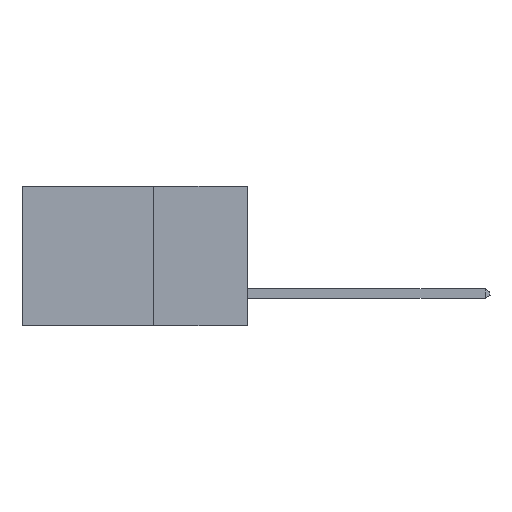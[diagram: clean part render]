
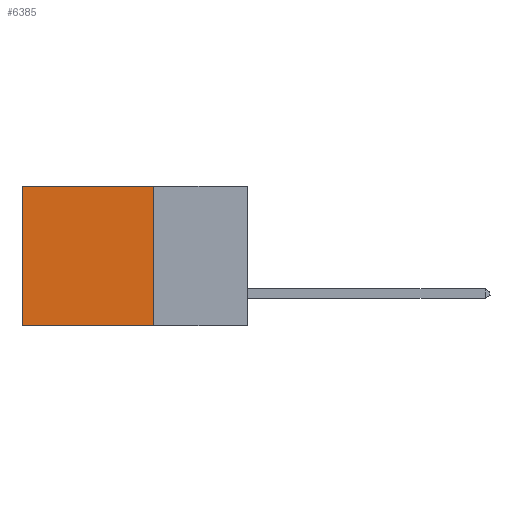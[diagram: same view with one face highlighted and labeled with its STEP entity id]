
A CAD part, left-side view. The second image highlights one B-rep face of the part: STEP entity #6385.
In plain terms, the highlighted planar face has unit normal (-1, 0, 0).
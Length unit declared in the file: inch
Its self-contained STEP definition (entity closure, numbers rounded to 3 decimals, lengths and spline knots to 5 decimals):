
#765 = ORIENTED_EDGE ( 'NONE', *, *, #7587, .F. ) ;
#781 = CARTESIAN_POINT ( 'NONE',  ( 0.298, 0.6, 0. ) ) ;
#1772 = LINE ( 'NONE', #2272, #2095 ) ;
#1887 = DIRECTION ( 'NONE',  ( 1., 0., 0. ) ) ;
#1901 = ORIENTED_EDGE ( 'NONE', *, *, #11786, .T. ) ;
#1933 = DIRECTION ( 'NONE',  ( 0., 0., -1. ) ) ;
#1983 = LINE ( 'NONE', #12808, #10273 ) ;
#2095 = VECTOR ( 'NONE', #10587, 39.37008 ) ;
#2272 = CARTESIAN_POINT ( 'NONE',  ( 0.298, 0.25, 0. ) ) ;
#2863 = AXIS2_PLACEMENT_3D ( 'NONE', #11199, #1887, #1933 ) ;
#2880 = CARTESIAN_POINT ( 'NONE',  ( 0.298, 0.25, -0.37 ) ) ;
#3035 = CARTESIAN_POINT ( 'NONE',  ( 0.298, 0.25, -0.37 ) ) ;
#3577 = CARTESIAN_POINT ( 'NONE',  ( 0.298, 0.6, -0.37 ) ) ;
#3998 = PLANE ( 'NONE',  #2863 ) ;
#4485 = DIRECTION ( 'NONE',  ( 0., 1., 0. ) ) ;
#4574 = VERTEX_POINT ( 'NONE', #5462 ) ;
#4881 = EDGE_LOOP ( 'NONE', ( #1901, #8925, #765, #7306 ) ) ;
#5462 = CARTESIAN_POINT ( 'NONE',  ( 0.298, 0.6, 0. ) ) ;
#5832 = EDGE_CURVE ( 'NONE', #10118, #4574, #1983, .T. ) ;
#5846 = DIRECTION ( 'NONE',  ( 0., 1., 0. ) ) ;
#5921 = VERTEX_POINT ( 'NONE', #3577 ) ;
#6385 = ADVANCED_FACE ( 'NONE', ( #7157 ), #3998, .F. ) ;
#7157 = FACE_OUTER_BOUND ( 'NONE', #4881, .T. ) ;
#7306 = ORIENTED_EDGE ( 'NONE', *, *, #5832, .T. ) ;
#7587 = EDGE_CURVE ( 'NONE', #10118, #10417, #1772, .T. ) ;
#7695 = LINE ( 'NONE', #2880, #10621 ) ;
#8031 = DIRECTION ( 'NONE',  ( 0., 0., -1. ) ) ;
#8925 = ORIENTED_EDGE ( 'NONE', *, *, #10825, .F. ) ;
#9440 = CARTESIAN_POINT ( 'NONE',  ( 0.298, 0.25, 0. ) ) ;
#9574 = VECTOR ( 'NONE', #8031, 39.37008 ) ;
#10118 = VERTEX_POINT ( 'NONE', #9440 ) ;
#10273 = VECTOR ( 'NONE', #4485, 39.37008 ) ;
#10417 = VERTEX_POINT ( 'NONE', #3035 ) ;
#10587 = DIRECTION ( 'NONE',  ( 0., 0., -1. ) ) ;
#10621 = VECTOR ( 'NONE', #5846, 39.37008 ) ;
#10825 = EDGE_CURVE ( 'NONE', #10417, #5921, #7695, .T. ) ;
#11199 = CARTESIAN_POINT ( 'NONE',  ( 0.298, 0.25, 0. ) ) ;
#11786 = EDGE_CURVE ( 'NONE', #4574, #5921, #12361, .T. ) ;
#12361 = LINE ( 'NONE', #781, #9574 ) ;
#12808 = CARTESIAN_POINT ( 'NONE',  ( 0.298, 0.25, 0. ) ) ;
